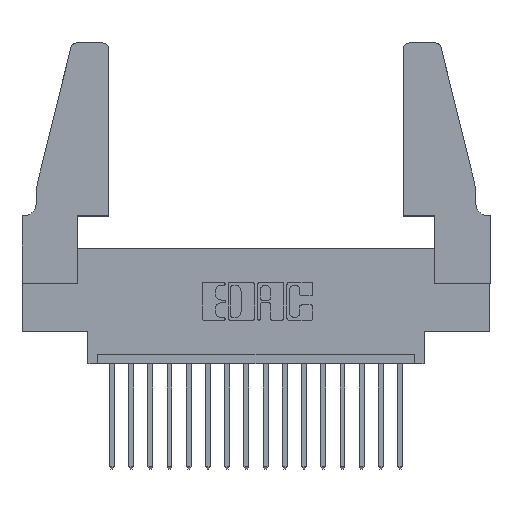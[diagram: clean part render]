
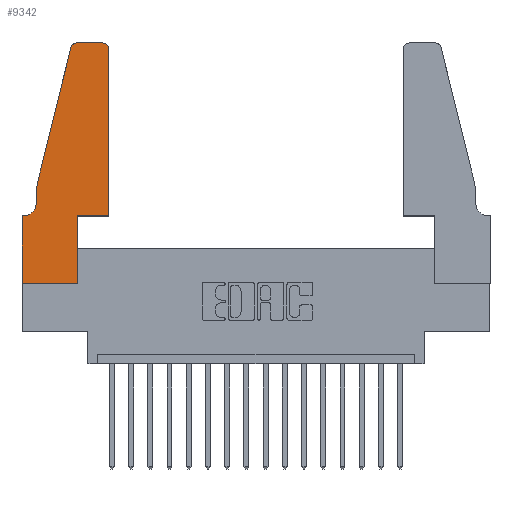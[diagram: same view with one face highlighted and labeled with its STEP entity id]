
A CAD part, top view. The second image highlights one B-rep face of the part: STEP entity #9342.
In plain terms, the highlighted planar face has unit normal (0, 0, 1).
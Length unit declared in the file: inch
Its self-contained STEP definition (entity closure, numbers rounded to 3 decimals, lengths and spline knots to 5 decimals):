
#11 = CARTESIAN_POINT ( 'NONE',  ( 0.2865, 0., 0.37 ) ) ;
#400 = EDGE_CURVE ( 'NONE', #3958, #1507, #2045, .T. ) ;
#401 = CARTESIAN_POINT ( 'NONE',  ( 0., 0.35, 0.37 ) ) ;
#604 = ORIENTED_EDGE ( 'NONE', *, *, #11476, .T. ) ;
#896 = ORIENTED_EDGE ( 'NONE', *, *, #7324, .T. ) ;
#1372 = CARTESIAN_POINT ( 'NONE',  ( 0.0755, 0.5, 0.37 ) ) ;
#1507 = VERTEX_POINT ( 'NONE', #11575 ) ;
#1617 = LINE ( 'NONE', #15665, #8546 ) ;
#1634 = CARTESIAN_POINT ( 'NONE',  ( 0.4205, 1.22, 0.37 ) ) ;
#1801 = VECTOR ( 'NONE', #11354, 39.37008 ) ;
#1830 = CARTESIAN_POINT ( 'NONE',  ( 0.4505, 0.35, 0.37 ) ) ;
#1876 = CARTESIAN_POINT ( 'NONE',  ( 0.0755, 0.5, 0.37 ) ) ;
#1898 = EDGE_CURVE ( 'NONE', #12484, #3918, #7218, .T. ) ;
#2045 = LINE ( 'NONE', #1876, #13701 ) ;
#2188 = VERTEX_POINT ( 'NONE', #6480 ) ;
#2482 = CARTESIAN_POINT ( 'NONE',  ( 0.284, 1.22, 0.37 ) ) ;
#2549 = PLANE ( 'NONE',  #6479 ) ;
#2606 = VERTEX_POINT ( 'NONE', #10820 ) ;
#2892 = DIRECTION ( 'NONE',  ( -1., 0., 0. ) ) ;
#2897 = EDGE_CURVE ( 'NONE', #8151, #4419, #9960, .T. ) ;
#3031 = CARTESIAN_POINT ( 'NONE',  ( 0.4505, 0.35, 0.37 ) ) ;
#3074 = DIRECTION ( 'NONE',  ( 1., 0., 0. ) ) ;
#3166 = CARTESIAN_POINT ( 'NONE',  ( 0.0755, 0.35, 0.37 ) ) ;
#3192 = CARTESIAN_POINT ( 'NONE',  ( 0.2865, 0.35, 0.37 ) ) ;
#3194 = VECTOR ( 'NONE', #8208, 39.37008 ) ;
#3386 = ORIENTED_EDGE ( 'NONE', *, *, #2897, .T. ) ;
#3501 = CARTESIAN_POINT ( 'NONE',  ( 0.4505, 0.35, 0.37 ) ) ;
#3884 = DIRECTION ( 'NONE',  ( 0., 0., -1. ) ) ;
#3915 = EDGE_CURVE ( 'NONE', #2188, #3958, #7336, .T. ) ;
#3918 = VERTEX_POINT ( 'NONE', #11 ) ;
#3958 = VERTEX_POINT ( 'NONE', #10860 ) ;
#4093 = EDGE_CURVE ( 'NONE', #14714, #15605, #15095, .T. ) ;
#4419 = VERTEX_POINT ( 'NONE', #3501 ) ;
#4951 = AXIS2_PLACEMENT_3D ( 'NONE', #1634, #11288, #3074 ) ;
#4967 = LINE ( 'NONE', #14486, #13563 ) ;
#5124 = CARTESIAN_POINT ( 'NONE',  ( 0., 0., 0.37 ) ) ;
#5654 = FACE_OUTER_BOUND ( 'NONE', #17413, .T. ) ;
#6032 = EDGE_CURVE ( 'NONE', #2606, #17851, #11564, .T. ) ;
#6033 = ORIENTED_EDGE ( 'NONE', *, *, #4093, .T. ) ;
#6479 = AXIS2_PLACEMENT_3D ( 'NONE', #11005, #6753, #6811 ) ;
#6480 = CARTESIAN_POINT ( 'NONE',  ( 0.25487, 1.22718, 0.37 ) ) ;
#6521 = DIRECTION ( 'NONE',  ( 0., 0., 1. ) ) ;
#6753 = DIRECTION ( 'NONE',  ( 0., 0., 1. ) ) ;
#6811 = DIRECTION ( 'NONE',  ( 1., 0., 0. ) ) ;
#6977 = ORIENTED_EDGE ( 'NONE', *, *, #7057, .T. ) ;
#7057 = EDGE_CURVE ( 'NONE', #9493, #2188, #7876, .T. ) ;
#7091 = EDGE_CURVE ( 'NONE', #1507, #14714, #11977, .T. ) ;
#7218 = LINE ( 'NONE', #5124, #9354 ) ;
#7324 = EDGE_CURVE ( 'NONE', #4419, #2606, #11089, .T. ) ;
#7336 = LINE ( 'NONE', #1372, #3194 ) ;
#7815 = DIRECTION ( 'NONE',  ( 0., -1., 0. ) ) ;
#7876 = CIRCLE ( 'NONE', #13708, 0.03 ) ;
#8151 = VERTEX_POINT ( 'NONE', #3192 ) ;
#8208 = DIRECTION ( 'NONE',  ( -0.239, -0.971, 0. ) ) ;
#8546 = VECTOR ( 'NONE', #8816, 39.37008 ) ;
#8816 = DIRECTION ( 'NONE',  ( -1., 0., 0. ) ) ;
#8948 = DIRECTION ( 'NONE',  ( 0., 1., 0. ) ) ;
#9342 = ADVANCED_FACE ( 'NONE', ( #5654 ), #2549, .T. ) ;
#9354 = VECTOR ( 'NONE', #17354, 39.37008 ) ;
#9493 = VERTEX_POINT ( 'NONE', #12656 ) ;
#9505 = VECTOR ( 'NONE', #7815, 39.37008 ) ;
#9752 = VECTOR ( 'NONE', #14449, 39.37008 ) ;
#9960 = LINE ( 'NONE', #1830, #9752 ) ;
#10139 = LINE ( 'NONE', #14809, #9505 ) ;
#10277 = ORIENTED_EDGE ( 'NONE', *, *, #1898, .T. ) ;
#10820 = CARTESIAN_POINT ( 'NONE',  ( 0.4505, 1.22, 0.37 ) ) ;
#10860 = CARTESIAN_POINT ( 'NONE',  ( 0.0755, 0.5, 0.37 ) ) ;
#11005 = CARTESIAN_POINT ( 'NONE',  ( 0., 0.35, 0.37 ) ) ;
#11089 = LINE ( 'NONE', #3031, #1801 ) ;
#11276 = AXIS2_PLACEMENT_3D ( 'NONE', #11370, #3884, #11944 ) ;
#11288 = DIRECTION ( 'NONE',  ( 0., 0., 1. ) ) ;
#11354 = DIRECTION ( 'NONE',  ( 0., 1., 0. ) ) ;
#11370 = CARTESIAN_POINT ( 'NONE',  ( 0.0055, 0.42, 0.37 ) ) ;
#11476 = EDGE_CURVE ( 'NONE', #17851, #9493, #1617, .T. ) ;
#11564 = CIRCLE ( 'NONE', #4951, 0.03 ) ;
#11575 = CARTESIAN_POINT ( 'NONE',  ( 0.0755, 0.42, 0.37 ) ) ;
#11652 = ORIENTED_EDGE ( 'NONE', *, *, #7091, .T. ) ;
#11790 = DIRECTION ( 'NONE',  ( 0., -1., 0. ) ) ;
#11944 = DIRECTION ( 'NONE',  ( -1., 0., 0. ) ) ;
#11977 = CIRCLE ( 'NONE', #11276, 0.07 ) ;
#12484 = VERTEX_POINT ( 'NONE', #13192 ) ;
#12492 = VECTOR ( 'NONE', #2892, 39.37008 ) ;
#12656 = CARTESIAN_POINT ( 'NONE',  ( 0.284, 1.25, 0.37 ) ) ;
#13192 = CARTESIAN_POINT ( 'NONE',  ( 0., 0., 0.37 ) ) ;
#13405 = CARTESIAN_POINT ( 'NONE',  ( 0.4205, 1.25, 0.37 ) ) ;
#13563 = VECTOR ( 'NONE', #8948, 39.37008 ) ;
#13612 = ORIENTED_EDGE ( 'NONE', *, *, #6032, .T. ) ;
#13701 = VECTOR ( 'NONE', #11790, 39.37008 ) ;
#13708 = AXIS2_PLACEMENT_3D ( 'NONE', #2482, #6521, #16131 ) ;
#13733 = ORIENTED_EDGE ( 'NONE', *, *, #3915, .T. ) ;
#14436 = ORIENTED_EDGE ( 'NONE', *, *, #16495, .T. ) ;
#14449 = DIRECTION ( 'NONE',  ( 1., 0., 0. ) ) ;
#14486 = CARTESIAN_POINT ( 'NONE',  ( 0.2865, 0.35, 0.37 ) ) ;
#14714 = VERTEX_POINT ( 'NONE', #15318 ) ;
#14809 = CARTESIAN_POINT ( 'NONE',  ( 0., 0., 0.37 ) ) ;
#14898 = EDGE_CURVE ( 'NONE', #15605, #12484, #10139, .T. ) ;
#15095 = LINE ( 'NONE', #3166, #12492 ) ;
#15318 = CARTESIAN_POINT ( 'NONE',  ( 0.0055, 0.35, 0.37 ) ) ;
#15585 = ORIENTED_EDGE ( 'NONE', *, *, #400, .T. ) ;
#15605 = VERTEX_POINT ( 'NONE', #401 ) ;
#15665 = CARTESIAN_POINT ( 'NONE',  ( 0.2605, 1.25, 0.37 ) ) ;
#16131 = DIRECTION ( 'NONE',  ( 1., 0., 0. ) ) ;
#16167 = ORIENTED_EDGE ( 'NONE', *, *, #14898, .T. ) ;
#16495 = EDGE_CURVE ( 'NONE', #3918, #8151, #4967, .T. ) ;
#17354 = DIRECTION ( 'NONE',  ( 1., 0., 0. ) ) ;
#17413 = EDGE_LOOP ( 'NONE', ( #604, #6977, #13733, #15585, #11652, #6033, #16167, #10277, #14436, #3386, #896, #13612 ) ) ;
#17851 = VERTEX_POINT ( 'NONE', #13405 ) ;
